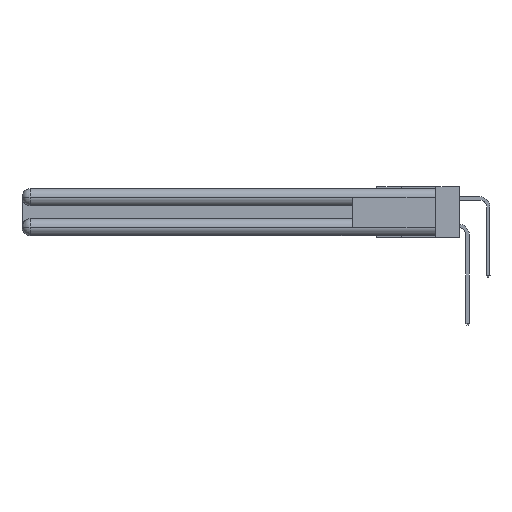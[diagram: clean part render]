
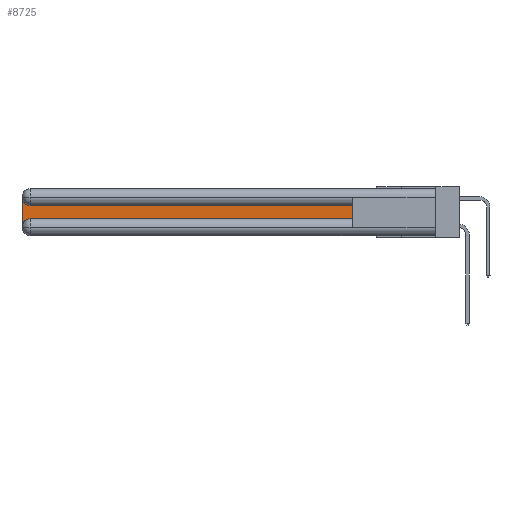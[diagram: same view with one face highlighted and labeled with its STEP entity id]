
A CAD part, left-side view. The second image highlights one B-rep face of the part: STEP entity #8725.
In plain terms, the highlighted planar face has unit normal (-1, 0, 0).
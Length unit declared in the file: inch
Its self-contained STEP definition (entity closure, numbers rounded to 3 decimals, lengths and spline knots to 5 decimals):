
#129 = DIRECTION ( 'NONE',  ( 0., 0., -1. ) ) ;
#225 = DIRECTION ( 'NONE',  ( 1., 0., 0. ) ) ;
#649 = DIRECTION ( 'NONE',  ( 0., 0., -1. ) ) ;
#3156 = VECTOR ( 'NONE', #11901, 39.37008 ) ;
#3423 = ORIENTED_EDGE ( 'NONE', *, *, #17947, .T. ) ;
#3658 = ORIENTED_EDGE ( 'NONE', *, *, #18309, .T. ) ;
#3854 = ORIENTED_EDGE ( 'NONE', *, *, #4074, .T. ) ;
#4074 = EDGE_CURVE ( 'NONE', #7660, #22126, #8887, .T. ) ;
#4150 = CIRCLE ( 'NONE', #6082, 0.06 ) ;
#4397 = LINE ( 'NONE', #22028, #23919 ) ;
#5090 = EDGE_LOOP ( 'NONE', ( #3423, #3854, #13081, #3658, #22896, #9248 ) ) ;
#5526 = DIRECTION ( 'NONE',  ( 1., 0., 0. ) ) ;
#6082 = AXIS2_PLACEMENT_3D ( 'NONE', #21083, #5526, #649 ) ;
#6117 = CARTESIAN_POINT ( 'NONE',  ( 0.075, 0.6, -0.2175 ) ) ;
#6645 = FACE_OUTER_BOUND ( 'NONE', #5090, .T. ) ;
#7660 = VERTEX_POINT ( 'NONE', #23517 ) ;
#8725 = ADVANCED_FACE ( 'NONE', ( #6645 ), #17462, .F. ) ;
#8766 = LINE ( 'NONE', #9131, #27933 ) ;
#8887 = CIRCLE ( 'NONE', #27530, 0.06 ) ;
#9131 = CARTESIAN_POINT ( 'NONE',  ( 0.075, 0.6, -0.2175 ) ) ;
#9248 = ORIENTED_EDGE ( 'NONE', *, *, #27353, .T. ) ;
#11529 = LINE ( 'NONE', #18333, #16208 ) ;
#11901 = DIRECTION ( 'NONE',  ( 0., 0., 1. ) ) ;
#12898 = DIRECTION ( 'NONE',  ( 0., 0., -1. ) ) ;
#13081 = ORIENTED_EDGE ( 'NONE', *, *, #23358, .T. ) ;
#13190 = VERTEX_POINT ( 'NONE', #20321 ) ;
#13550 = DIRECTION ( 'NONE',  ( 0., -1., 0. ) ) ;
#13842 = DIRECTION ( 'NONE',  ( 0., 1., 0. ) ) ;
#15210 = VERTEX_POINT ( 'NONE', #15566 ) ;
#15566 = CARTESIAN_POINT ( 'NONE',  ( 0.075, 0.6, -0.1225 ) ) ;
#16208 = VECTOR ( 'NONE', #13842, 39.37008 ) ;
#17462 = PLANE ( 'NONE',  #21669 ) ;
#17947 = EDGE_CURVE ( 'NONE', #15210, #7660, #11529, .T. ) ;
#18309 = EDGE_CURVE ( 'NONE', #28357, #13190, #4150, .T. ) ;
#18333 = CARTESIAN_POINT ( 'NONE',  ( 0.075, 0.6, -0.1225 ) ) ;
#18441 = DIRECTION ( 'NONE',  ( 0., 0., -1. ) ) ;
#18819 = CARTESIAN_POINT ( 'NONE',  ( 0.075, 0.6, -0.2175 ) ) ;
#19709 = EDGE_CURVE ( 'NONE', #13190, #27548, #8766, .T. ) ;
#20321 = CARTESIAN_POINT ( 'NONE',  ( 0.075, 2.94, -0.2175 ) ) ;
#20835 = CARTESIAN_POINT ( 'NONE',  ( 0.075, 2.94, -0.0625 ) ) ;
#21083 = CARTESIAN_POINT ( 'NONE',  ( 0.075, 2.94, -0.2775 ) ) ;
#21487 = CARTESIAN_POINT ( 'NONE',  ( 0.075, 3., -0.0625 ) ) ;
#21669 = AXIS2_PLACEMENT_3D ( 'NONE', #24610, #29194, #129 ) ;
#21836 = CARTESIAN_POINT ( 'NONE',  ( 0.075, 3., -0.2775 ) ) ;
#22028 = CARTESIAN_POINT ( 'NONE',  ( 0.075, 3., -0.2175 ) ) ;
#22126 = VERTEX_POINT ( 'NONE', #21487 ) ;
#22896 = ORIENTED_EDGE ( 'NONE', *, *, #19709, .T. ) ;
#23358 = EDGE_CURVE ( 'NONE', #22126, #28357, #4397, .T. ) ;
#23517 = CARTESIAN_POINT ( 'NONE',  ( 0.075, 2.94, -0.1225 ) ) ;
#23919 = VECTOR ( 'NONE', #12898, 39.37008 ) ;
#24610 = CARTESIAN_POINT ( 'NONE',  ( 0.075, 3., -0.1225 ) ) ;
#26542 = LINE ( 'NONE', #18819, #3156 ) ;
#27353 = EDGE_CURVE ( 'NONE', #27548, #15210, #26542, .T. ) ;
#27530 = AXIS2_PLACEMENT_3D ( 'NONE', #20835, #225, #18441 ) ;
#27548 = VERTEX_POINT ( 'NONE', #6117 ) ;
#27933 = VECTOR ( 'NONE', #13550, 39.37008 ) ;
#28357 = VERTEX_POINT ( 'NONE', #21836 ) ;
#29194 = DIRECTION ( 'NONE',  ( 1., 0., 0. ) ) ;
